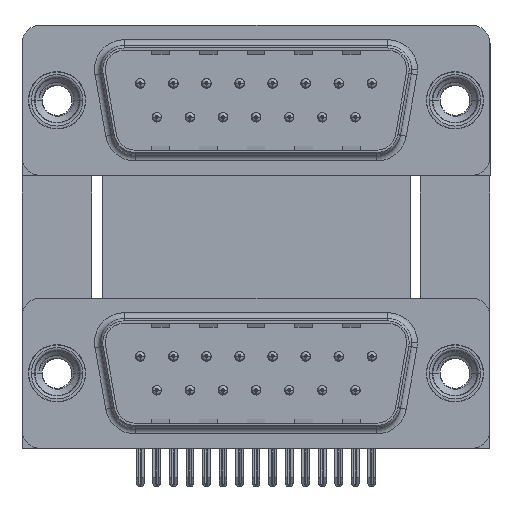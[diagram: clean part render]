
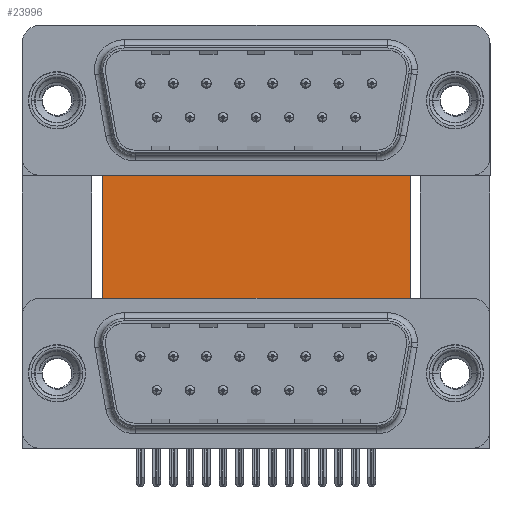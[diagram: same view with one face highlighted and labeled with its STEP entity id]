
A CAD part, top view. The second image highlights one B-rep face of the part: STEP entity #23996.
In plain terms, the highlighted planar face has unit normal (0, 0, 1).
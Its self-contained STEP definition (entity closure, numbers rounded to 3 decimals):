
#598 = ORIENTED_EDGE ( 'NONE', *, *, #7206, .F. ) ;
#1087 = VERTEX_POINT ( 'NONE', #12383 ) ;
#1610 = PLANE ( 'NONE',  #2117 ) ;
#2117 = AXIS2_PLACEMENT_3D ( 'NONE', #18897, #13824, #6844 ) ;
#2386 = DIRECTION ( 'NONE',  ( 0., -1., 0. ) ) ;
#3818 = CARTESIAN_POINT ( 'NONE',  ( 29.58, -3.735, -12. ) ) ;
#4235 = VECTOR ( 'NONE', #20255, 1000. ) ;
#4429 = VECTOR ( 'NONE', #2386, 1000. ) ;
#4455 = FACE_OUTER_BOUND ( 'NONE', #7163, .T. ) ;
#6795 = LINE ( 'NONE', #9168, #11090 ) ;
#6844 = DIRECTION ( 'NONE',  ( -1., 0., 0. ) ) ;
#7163 = EDGE_LOOP ( 'NONE', ( #25950, #26528, #598, #20288 ) ) ;
#7206 = EDGE_CURVE ( 'NONE', #29149, #7862, #26983, .T. ) ;
#7301 = CARTESIAN_POINT ( 'NONE',  ( 3.79, 16.585, -12. ) ) ;
#7318 = CARTESIAN_POINT ( 'NONE',  ( 3.79, 16.585, -12. ) ) ;
#7862 = VERTEX_POINT ( 'NONE', #28007 ) ;
#9168 = CARTESIAN_POINT ( 'NONE',  ( 3.79, -3.735, -12. ) ) ;
#9477 = DIRECTION ( 'NONE',  ( 1., 0., 0. ) ) ;
#10171 = VECTOR ( 'NONE', #22613, 1000. ) ;
#10579 = CARTESIAN_POINT ( 'NONE',  ( 3.79, 16.585, -12. ) ) ;
#11090 = VECTOR ( 'NONE', #9477, 1000. ) ;
#12329 = CARTESIAN_POINT ( 'NONE',  ( 29.58, 16.585, -12. ) ) ;
#12383 = CARTESIAN_POINT ( 'NONE',  ( 3.79, -3.735, -12. ) ) ;
#13824 = DIRECTION ( 'NONE',  ( 0., 0., -1. ) ) ;
#15156 = LINE ( 'NONE', #7301, #4429 ) ;
#17043 = EDGE_CURVE ( 'NONE', #29149, #1087, #15156, .T. ) ;
#17529 = LINE ( 'NONE', #12329, #10171 ) ;
#17932 = VERTEX_POINT ( 'NONE', #3818 ) ;
#18877 = EDGE_CURVE ( 'NONE', #1087, #17932, #6795, .T. ) ;
#18897 = CARTESIAN_POINT ( 'NONE',  ( 3.79, 16.585, -12. ) ) ;
#20255 = DIRECTION ( 'NONE',  ( 1., 0., 0. ) ) ;
#20288 = ORIENTED_EDGE ( 'NONE', *, *, #17043, .T. ) ;
#22613 = DIRECTION ( 'NONE',  ( 0., -1., 0. ) ) ;
#23996 = ADVANCED_FACE ( 'NONE', ( #4455 ), #1610, .F. ) ;
#25950 = ORIENTED_EDGE ( 'NONE', *, *, #18877, .T. ) ;
#26528 = ORIENTED_EDGE ( 'NONE', *, *, #30181, .F. ) ;
#26983 = LINE ( 'NONE', #10579, #4235 ) ;
#28007 = CARTESIAN_POINT ( 'NONE',  ( 29.58, 16.585, -12. ) ) ;
#29149 = VERTEX_POINT ( 'NONE', #7318 ) ;
#30181 = EDGE_CURVE ( 'NONE', #7862, #17932, #17529, .T. ) ;
